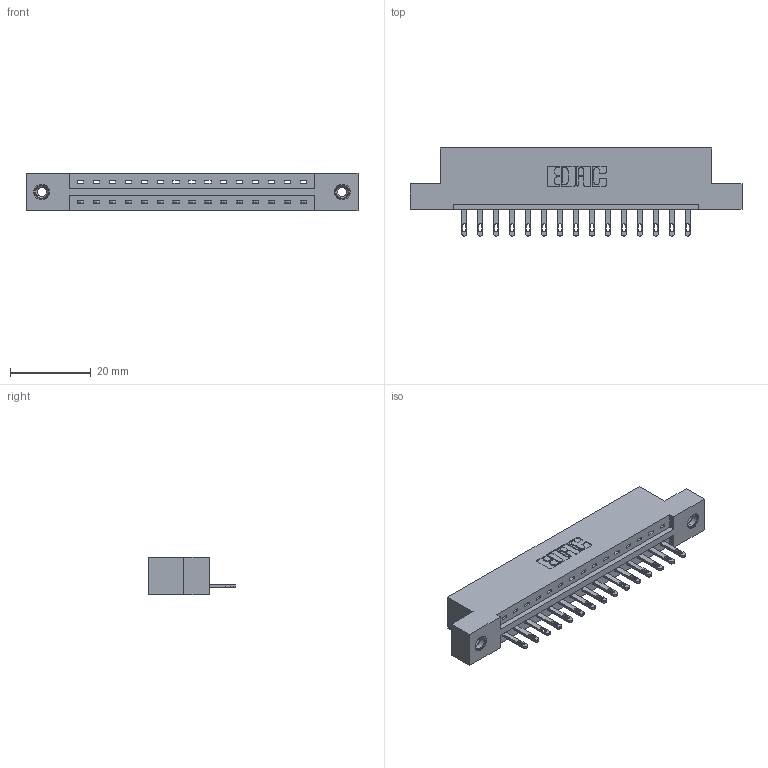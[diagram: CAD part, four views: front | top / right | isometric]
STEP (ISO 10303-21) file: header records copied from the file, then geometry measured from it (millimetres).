
FILE_DESCRIPTION (( 'STEP AP203' ), '1' );
FILE_NAME ('887-015-500-108.STEP', '2020-09-20T17:01:55', ( '' ), ( '' ), 'SwSTEP 2.0', 'SolidWorks 2020', '' );
FILE_SCHEMA (( 'CONFIG_CONTROL_DESIGN' ));
Length unit declared in the file: inch
Products named in the file (4): 837 Part_Flush Mounting Lugs - 0.156 Dia-TI; 887-015-500-108; 345-292-001_345-293-100; 345-250-001_345-250-003-102
Assembly tree (18 placements, depth 2):
  887-015-500-108
    837 Part_Flush Mounting Lugs - 0.156 Dia-TI
    345-292-001_345-293-100  x15
    345-250-001_345-250-003-102  x2
Bounding box: 82.45 x 21.85 x 9.4 mm (x, y, z)
Volume: 8234 mm3; surface area: 8423.5 mm2
Topology: 18 solids, 18 shells, 1044 faces, 3147 edges, 2090 vertices
Faces by surface type: plane 702, cylinder 326, cone 12, torus 4
Entity records: 15758 total; most frequent: CARTESIAN_POINT 2722, ORIENTED_EDGE 2666, DIRECTION 2381, EDGE_CURVE 1333, LINE 1181, VECTOR 1181, VERTEX_POINT 884, AXIS2_PLACEMENT_3D 600
